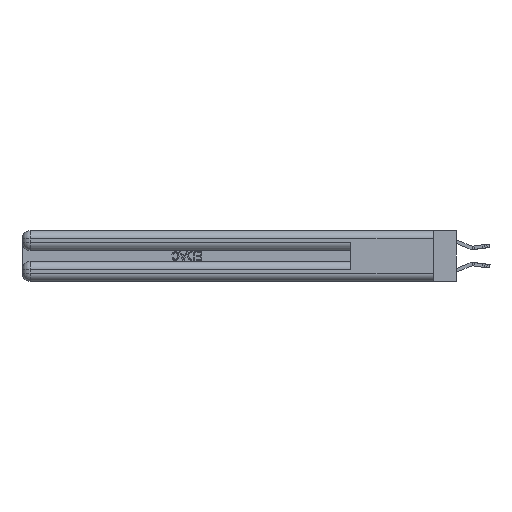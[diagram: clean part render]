
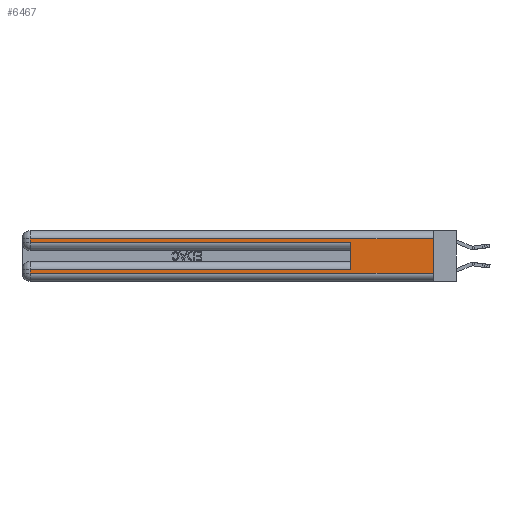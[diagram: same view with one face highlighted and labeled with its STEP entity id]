
A CAD part, left-side view. The second image highlights one B-rep face of the part: STEP entity #6467.
In plain terms, the highlighted planar face has unit normal (-1, 0, 0).
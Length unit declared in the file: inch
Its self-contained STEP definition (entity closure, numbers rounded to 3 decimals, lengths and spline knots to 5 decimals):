
#48 = LINE ( 'NONE', #2827, #31057 ) ;
#54 = DIRECTION ( 'NONE',  ( 0., 1., 0. ) ) ;
#305 = DIRECTION ( 'NONE',  ( 0., -1., 0. ) ) ;
#437 = CARTESIAN_POINT ( 'NONE',  ( 0., 0., 0.31 ) ) ;
#1249 = CARTESIAN_POINT ( 'NONE',  ( 0., 0., 0.31 ) ) ;
#1261 = LINE ( 'NONE', #7830, #15561 ) ;
#1328 = VECTOR ( 'NONE', #54, 39.37008 ) ;
#1733 = ORIENTED_EDGE ( 'NONE', *, *, #31048, .T. ) ;
#2031 = EDGE_LOOP ( 'NONE', ( #21050, #12749, #20654, #24512, #20821, #18811, #6697, #1733 ) ) ;
#2033 = CARTESIAN_POINT ( 'NONE',  ( 0., 2.94, 0.285 ) ) ;
#2467 = EDGE_CURVE ( 'NONE', #29361, #27946, #48, .T. ) ;
#2827 = CARTESIAN_POINT ( 'NONE',  ( 0., 0.6, 0.145 ) ) ;
#2850 = CARTESIAN_POINT ( 'NONE',  ( 0., 0., 0.06 ) ) ;
#3155 = DIRECTION ( 'NONE',  ( 0., 1., 0. ) ) ;
#3193 = EDGE_CURVE ( 'NONE', #29361, #6934, #22244, .T. ) ;
#4095 = DIRECTION ( 'NONE',  ( 0., -1., 0. ) ) ;
#6467 = ADVANCED_FACE ( 'NONE', ( #31372 ), #10262, .F. ) ;
#6697 = ORIENTED_EDGE ( 'NONE', *, *, #24312, .T. ) ;
#6934 = VERTEX_POINT ( 'NONE', #25890 ) ;
#7507 = VERTEX_POINT ( 'NONE', #33319 ) ;
#7830 = CARTESIAN_POINT ( 'NONE',  ( 0., 2.94, 0.37 ) ) ;
#9259 = DIRECTION ( 'NONE',  ( 0., 0., -1. ) ) ;
#10262 = PLANE ( 'NONE',  #31825 ) ;
#11039 = CARTESIAN_POINT ( 'NONE',  ( 0., 0., 0.085 ) ) ;
#11433 = LINE ( 'NONE', #22717, #17656 ) ;
#12152 = VECTOR ( 'NONE', #3155, 39.37008 ) ;
#12749 = ORIENTED_EDGE ( 'NONE', *, *, #26337, .T. ) ;
#12962 = DIRECTION ( 'NONE',  ( 0., 0., -1. ) ) ;
#13549 = VERTEX_POINT ( 'NONE', #1249 ) ;
#13813 = EDGE_CURVE ( 'NONE', #13549, #34363, #31992, .T. ) ;
#14720 = LINE ( 'NONE', #24442, #28863 ) ;
#15561 = VECTOR ( 'NONE', #26515, 39.37008 ) ;
#16823 = CARTESIAN_POINT ( 'NONE',  ( 0., 0.6, 0.285 ) ) ;
#17656 = VECTOR ( 'NONE', #4095, 39.37008 ) ;
#17838 = VECTOR ( 'NONE', #31625, 39.37008 ) ;
#18811 = ORIENTED_EDGE ( 'NONE', *, *, #3193, .T. ) ;
#19435 = EDGE_CURVE ( 'NONE', #24055, #25482, #1261, .T. ) ;
#20654 = ORIENTED_EDGE ( 'NONE', *, *, #19435, .T. ) ;
#20821 = ORIENTED_EDGE ( 'NONE', *, *, #2467, .F. ) ;
#20883 = LINE ( 'NONE', #437, #12152 ) ;
#21050 = ORIENTED_EDGE ( 'NONE', *, *, #13813, .F. ) ;
#21480 = VECTOR ( 'NONE', #9259, 39.37008 ) ;
#21567 = DIRECTION ( 'NONE',  ( 0., 0., 1. ) ) ;
#22244 = LINE ( 'NONE', #11039, #1328 ) ;
#22717 = CARTESIAN_POINT ( 'NONE',  ( 0., 0., 0.285 ) ) ;
#24055 = VERTEX_POINT ( 'NONE', #24120 ) ;
#24120 = CARTESIAN_POINT ( 'NONE',  ( 0., 2.94, 0.31 ) ) ;
#24312 = EDGE_CURVE ( 'NONE', #6934, #7507, #26866, .T. ) ;
#24442 = CARTESIAN_POINT ( 'NONE',  ( 0., 0., 0.06 ) ) ;
#24512 = ORIENTED_EDGE ( 'NONE', *, *, #30664, .T. ) ;
#25482 = VERTEX_POINT ( 'NONE', #2033 ) ;
#25890 = CARTESIAN_POINT ( 'NONE',  ( 0., 2.94, 0.085 ) ) ;
#26207 = CARTESIAN_POINT ( 'NONE',  ( 0., 0., 0.37 ) ) ;
#26337 = EDGE_CURVE ( 'NONE', #13549, #24055, #20883, .T. ) ;
#26515 = DIRECTION ( 'NONE',  ( 0., 0., -1. ) ) ;
#26866 = LINE ( 'NONE', #33289, #21480 ) ;
#27946 = VERTEX_POINT ( 'NONE', #16823 ) ;
#28863 = VECTOR ( 'NONE', #305, 39.37008 ) ;
#28899 = DIRECTION ( 'NONE',  ( 1., 0., 0. ) ) ;
#29361 = VERTEX_POINT ( 'NONE', #30824 ) ;
#30664 = EDGE_CURVE ( 'NONE', #25482, #27946, #11433, .T. ) ;
#30824 = CARTESIAN_POINT ( 'NONE',  ( 0., 0.6, 0.085 ) ) ;
#31048 = EDGE_CURVE ( 'NONE', #7507, #34363, #14720, .T. ) ;
#31057 = VECTOR ( 'NONE', #21567, 39.37008 ) ;
#31372 = FACE_OUTER_BOUND ( 'NONE', #2031, .T. ) ;
#31625 = DIRECTION ( 'NONE',  ( 0., 0., -1. ) ) ;
#31825 = AXIS2_PLACEMENT_3D ( 'NONE', #26207, #28899, #12962 ) ;
#31992 = LINE ( 'NONE', #34302, #17838 ) ;
#33289 = CARTESIAN_POINT ( 'NONE',  ( 0., 2.94, 0.37 ) ) ;
#33319 = CARTESIAN_POINT ( 'NONE',  ( 0., 2.94, 0.06 ) ) ;
#34302 = CARTESIAN_POINT ( 'NONE',  ( 0., 0., 0.37 ) ) ;
#34363 = VERTEX_POINT ( 'NONE', #2850 ) ;
